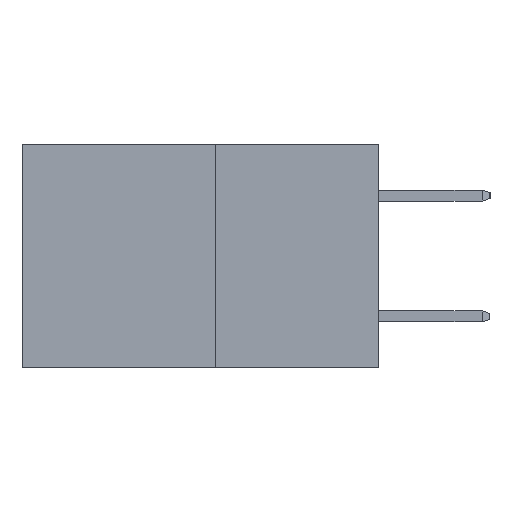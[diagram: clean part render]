
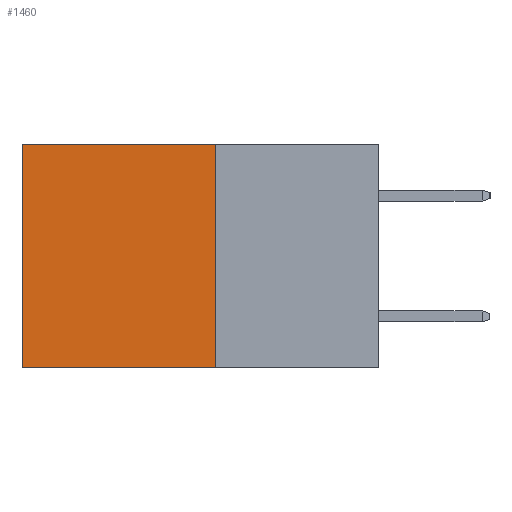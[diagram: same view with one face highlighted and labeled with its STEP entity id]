
A CAD part, left-side view. The second image highlights one B-rep face of the part: STEP entity #1460.
In plain terms, the highlighted planar face has unit normal (-1, 0, 0).
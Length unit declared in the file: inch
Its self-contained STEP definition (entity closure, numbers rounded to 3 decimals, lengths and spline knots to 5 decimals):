
#13 = LINE ( 'NONE', #4958, #7111 ) ;
#456 = CARTESIAN_POINT ( 'NONE',  ( 0.277, 0.59, 0. ) ) ;
#461 = DIRECTION ( 'NONE',  ( 0., 0., -1. ) ) ;
#526 = CARTESIAN_POINT ( 'NONE',  ( 0.277, 0.27, -0.37 ) ) ;
#936 = VECTOR ( 'NONE', #6963, 39.37008 ) ;
#965 = CARTESIAN_POINT ( 'NONE',  ( 0.277, 0.27, -0.37 ) ) ;
#1278 = DIRECTION ( 'NONE',  ( 0., 0., -1. ) ) ;
#1460 = ADVANCED_FACE ( 'NONE', ( #1900 ), #1915, .F. ) ;
#1900 = FACE_OUTER_BOUND ( 'NONE', #9276, .T. ) ;
#1915 = PLANE ( 'NONE',  #10411 ) ;
#3281 = VERTEX_POINT ( 'NONE', #456 ) ;
#3306 = EDGE_CURVE ( 'NONE', #3417, #3281, #10252, .T. ) ;
#3417 = VERTEX_POINT ( 'NONE', #11526 ) ;
#3787 = EDGE_CURVE ( 'NONE', #8290, #8461, #4231, .T. ) ;
#4231 = LINE ( 'NONE', #526, #5988 ) ;
#4302 = CARTESIAN_POINT ( 'NONE',  ( 0.277, 0.59, -0.37 ) ) ;
#4404 = DIRECTION ( 'NONE',  ( 0., 1., 0. ) ) ;
#4958 = CARTESIAN_POINT ( 'NONE',  ( 0.277, 0.27, -0.37 ) ) ;
#5068 = ORIENTED_EDGE ( 'NONE', *, *, #9160, .F. ) ;
#5988 = VECTOR ( 'NONE', #4404, 39.37008 ) ;
#6066 = CARTESIAN_POINT ( 'NONE',  ( 0.277, 0.27, 0. ) ) ;
#6177 = VECTOR ( 'NONE', #461, 39.37008 ) ;
#6963 = DIRECTION ( 'NONE',  ( 0., 1., 0. ) ) ;
#7025 = EDGE_CURVE ( 'NONE', #3281, #8461, #8521, .T. ) ;
#7106 = ORIENTED_EDGE ( 'NONE', *, *, #3787, .F. ) ;
#7111 = VECTOR ( 'NONE', #1278, 39.37008 ) ;
#7635 = ORIENTED_EDGE ( 'NONE', *, *, #3306, .T. ) ;
#8290 = VERTEX_POINT ( 'NONE', #965 ) ;
#8461 = VERTEX_POINT ( 'NONE', #10302 ) ;
#8521 = LINE ( 'NONE', #4302, #6177 ) ;
#9160 = EDGE_CURVE ( 'NONE', #3417, #8290, #13, .T. ) ;
#9276 = EDGE_LOOP ( 'NONE', ( #10931, #7106, #5068, #7635 ) ) ;
#10252 = LINE ( 'NONE', #6066, #936 ) ;
#10302 = CARTESIAN_POINT ( 'NONE',  ( 0.277, 0.59, -0.37 ) ) ;
#10411 = AXIS2_PLACEMENT_3D ( 'NONE', #10808, #10736, #10720 ) ;
#10720 = DIRECTION ( 'NONE',  ( 0., 0., -1. ) ) ;
#10736 = DIRECTION ( 'NONE',  ( 1., 0., 0. ) ) ;
#10808 = CARTESIAN_POINT ( 'NONE',  ( 0.277, 0.27, -0.37 ) ) ;
#10931 = ORIENTED_EDGE ( 'NONE', *, *, #7025, .T. ) ;
#11526 = CARTESIAN_POINT ( 'NONE',  ( 0.277, 0.27, 0. ) ) ;
